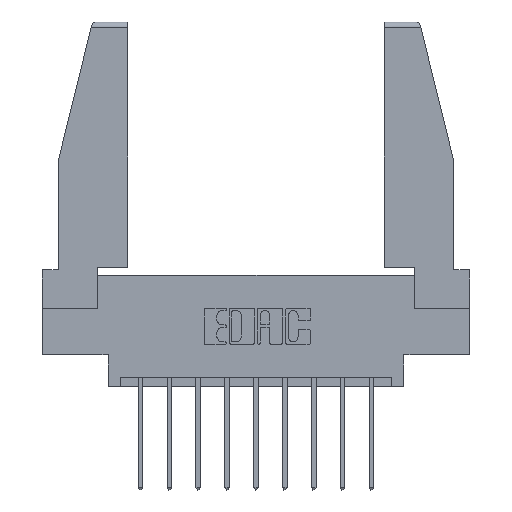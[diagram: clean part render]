
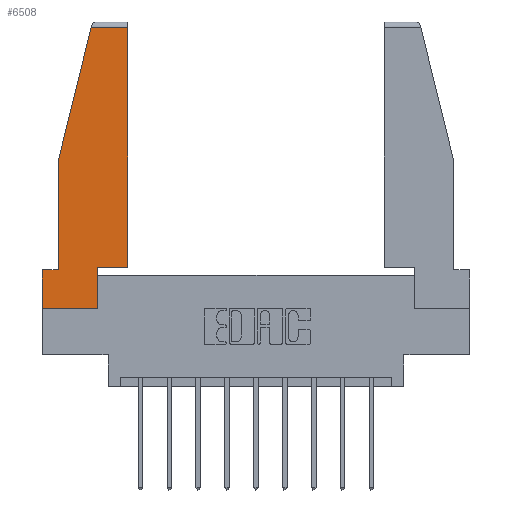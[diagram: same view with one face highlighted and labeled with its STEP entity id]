
A CAD part, top view. The second image highlights one B-rep face of the part: STEP entity #6508.
In plain terms, the highlighted planar face has unit normal (0, 0, 1).
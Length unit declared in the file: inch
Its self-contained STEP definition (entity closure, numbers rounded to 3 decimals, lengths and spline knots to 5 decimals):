
#411 = EDGE_CURVE ( 'NONE', #3429, #5769, #9034, .T. ) ;
#941 = LINE ( 'NONE', #9646, #11995 ) ;
#967 = VECTOR ( 'NONE', #1119, 39.37008 ) ;
#1119 = DIRECTION ( 'NONE',  ( 1., 0., 0. ) ) ;
#1238 = LINE ( 'NONE', #7818, #9789 ) ;
#1281 = EDGE_CURVE ( 'NONE', #3022, #3429, #3792, .T. ) ;
#1562 = DIRECTION ( 'NONE',  ( 0., 1., 0. ) ) ;
#1610 = LINE ( 'NONE', #3382, #8659 ) ;
#1677 = EDGE_LOOP ( 'NONE', ( #9368, #11028, #2945, #13766, #2894, #5326, #6237, #8068, #6985 ) ) ;
#1813 = VECTOR ( 'NONE', #1562, 39.37008 ) ;
#1926 = DIRECTION ( 'NONE',  ( -1., 0., 0. ) ) ;
#1956 = LINE ( 'NONE', #4509, #11839 ) ;
#2231 = CARTESIAN_POINT ( 'NONE',  ( 0.271, 1.55, 0. ) ) ;
#2533 = CARTESIAN_POINT ( 'NONE',  ( 0.297, 0., 0. ) ) ;
#2676 = CARTESIAN_POINT ( 'NONE',  ( 0., 0., 0. ) ) ;
#2894 = ORIENTED_EDGE ( 'NONE', *, *, #12084, .T. ) ;
#2945 = ORIENTED_EDGE ( 'NONE', *, *, #10668, .T. ) ;
#3022 = VERTEX_POINT ( 'NONE', #10460 ) ;
#3382 = CARTESIAN_POINT ( 'NONE',  ( 0., 0., 0. ) ) ;
#3429 = VERTEX_POINT ( 'NONE', #13172 ) ;
#3475 = LINE ( 'NONE', #2231, #12353 ) ;
#3585 = DIRECTION ( 'NONE',  ( 0., 0., 1. ) ) ;
#3792 = LINE ( 'NONE', #6545, #967 ) ;
#4250 = EDGE_CURVE ( 'NONE', #5769, #6833, #7412, .T. ) ;
#4277 = DIRECTION ( 'NONE',  ( -1., 0., 0. ) ) ;
#4509 = CARTESIAN_POINT ( 'NONE',  ( 0.297, 0., 0. ) ) ;
#5072 = CARTESIAN_POINT ( 'NONE',  ( 0., 1.52, 0. ) ) ;
#5326 = ORIENTED_EDGE ( 'NONE', *, *, #8305, .T. ) ;
#5356 = VERTEX_POINT ( 'NONE', #2533 ) ;
#5393 = CARTESIAN_POINT ( 'NONE',  ( 0., 0.21, 0. ) ) ;
#5769 = VERTEX_POINT ( 'NONE', #6695 ) ;
#5896 = EDGE_CURVE ( 'NONE', #5356, #3022, #1956, .T. ) ;
#6034 = CARTESIAN_POINT ( 'NONE',  ( 0.2636, 1.52, 0. ) ) ;
#6237 = ORIENTED_EDGE ( 'NONE', *, *, #12545, .T. ) ;
#6508 = ADVANCED_FACE ( 'NONE', ( #11660 ), #7791, .T. ) ;
#6545 = CARTESIAN_POINT ( 'NONE',  ( 0.297, 0.223, 0. ) ) ;
#6586 = DIRECTION ( 'NONE',  ( 0., -1., 0. ) ) ;
#6681 = CARTESIAN_POINT ( 'NONE',  ( 0., 0., 0. ) ) ;
#6695 = CARTESIAN_POINT ( 'NONE',  ( 0.461, 1.52, 0. ) ) ;
#6833 = VERTEX_POINT ( 'NONE', #6034 ) ;
#6888 = CARTESIAN_POINT ( 'NONE',  ( 0.461, 0.223, 0. ) ) ;
#6985 = ORIENTED_EDGE ( 'NONE', *, *, #1281, .T. ) ;
#7235 = VERTEX_POINT ( 'NONE', #12211 ) ;
#7412 = LINE ( 'NONE', #5072, #13266 ) ;
#7516 = CARTESIAN_POINT ( 'NONE',  ( 0.086, 0.8, 0. ) ) ;
#7519 = DIRECTION ( 'NONE',  ( -0.239, -0.971, 0. ) ) ;
#7625 = DIRECTION ( 'NONE',  ( 0., 1., 0. ) ) ;
#7791 = PLANE ( 'NONE',  #12002 ) ;
#7818 = CARTESIAN_POINT ( 'NONE',  ( 0., 0.21, 0. ) ) ;
#8068 = ORIENTED_EDGE ( 'NONE', *, *, #5896, .T. ) ;
#8305 = EDGE_CURVE ( 'NONE', #8679, #11421, #1238, .T. ) ;
#8659 = VECTOR ( 'NONE', #10737, 39.37008 ) ;
#8679 = VERTEX_POINT ( 'NONE', #5393 ) ;
#8959 = DIRECTION ( 'NONE',  ( 0., -1., 0. ) ) ;
#9034 = LINE ( 'NONE', #6888, #1813 ) ;
#9368 = ORIENTED_EDGE ( 'NONE', *, *, #411, .T. ) ;
#9646 = CARTESIAN_POINT ( 'NONE',  ( 0., 0.21, 0. ) ) ;
#9717 = VERTEX_POINT ( 'NONE', #10886 ) ;
#9789 = VECTOR ( 'NONE', #8959, 39.37008 ) ;
#10033 = VECTOR ( 'NONE', #6586, 39.37008 ) ;
#10299 = EDGE_CURVE ( 'NONE', #7235, #9717, #12363, .T. ) ;
#10460 = CARTESIAN_POINT ( 'NONE',  ( 0.297, 0.223, 0. ) ) ;
#10668 = EDGE_CURVE ( 'NONE', #6833, #7235, #3475, .T. ) ;
#10737 = DIRECTION ( 'NONE',  ( 1., 0., 0. ) ) ;
#10880 = DIRECTION ( 'NONE',  ( 1., 0., 0. ) ) ;
#10886 = CARTESIAN_POINT ( 'NONE',  ( 0.086, 0.21, 0. ) ) ;
#11028 = ORIENTED_EDGE ( 'NONE', *, *, #4250, .T. ) ;
#11421 = VERTEX_POINT ( 'NONE', #2676 ) ;
#11660 = FACE_OUTER_BOUND ( 'NONE', #1677, .T. ) ;
#11839 = VECTOR ( 'NONE', #7625, 39.37008 ) ;
#11995 = VECTOR ( 'NONE', #4277, 39.37008 ) ;
#12002 = AXIS2_PLACEMENT_3D ( 'NONE', #6681, #3585, #10880 ) ;
#12084 = EDGE_CURVE ( 'NONE', #9717, #8679, #941, .T. ) ;
#12211 = CARTESIAN_POINT ( 'NONE',  ( 0.086, 0.8, 0. ) ) ;
#12353 = VECTOR ( 'NONE', #7519, 39.37008 ) ;
#12363 = LINE ( 'NONE', #7516, #10033 ) ;
#12545 = EDGE_CURVE ( 'NONE', #11421, #5356, #1610, .T. ) ;
#13172 = CARTESIAN_POINT ( 'NONE',  ( 0.461, 0.223, 0. ) ) ;
#13266 = VECTOR ( 'NONE', #1926, 39.37008 ) ;
#13766 = ORIENTED_EDGE ( 'NONE', *, *, #10299, .T. ) ;
